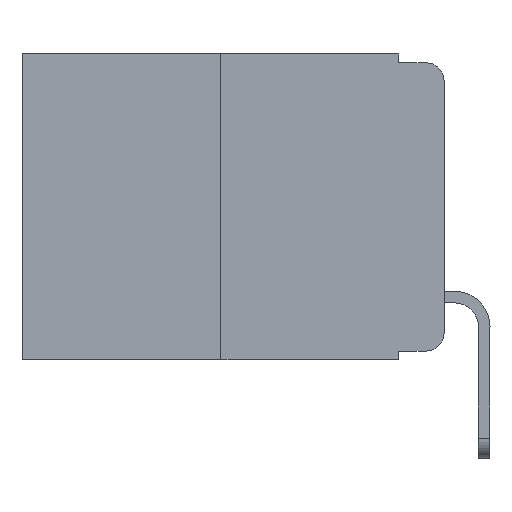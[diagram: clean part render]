
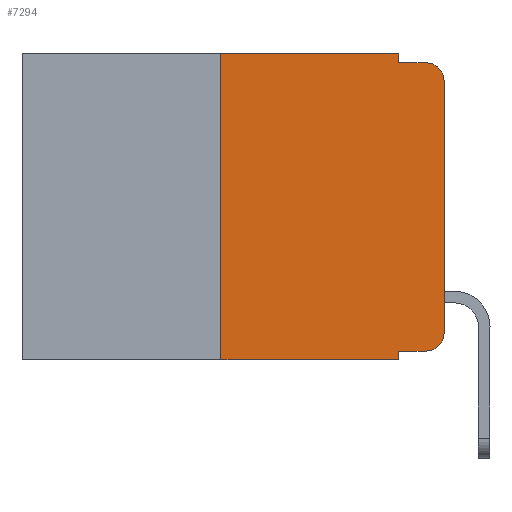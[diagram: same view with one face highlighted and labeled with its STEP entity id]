
A CAD part, left-side view. The second image highlights one B-rep face of the part: STEP entity #7294.
In plain terms, the highlighted planar face has unit normal (-1, 0, 0).
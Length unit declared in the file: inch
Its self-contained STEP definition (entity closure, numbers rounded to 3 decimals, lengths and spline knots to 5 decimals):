
#177 = ORIENTED_EDGE ( 'NONE', *, *, #3512, .F. ) ;
#372 = CARTESIAN_POINT ( 'NONE',  ( 0., 0.02, -0.01 ) ) ;
#486 = VECTOR ( 'NONE', #6335, 39.37008 ) ;
#684 = DIRECTION ( 'NONE',  ( 0., -1., 0. ) ) ;
#727 = FACE_OUTER_BOUND ( 'NONE', #8281, .T. ) ;
#996 = DIRECTION ( 'NONE',  ( 0., -1., 0. ) ) ;
#1347 = DIRECTION ( 'NONE',  ( 0., 0., -1. ) ) ;
#1359 = LINE ( 'NONE', #2402, #486 ) ;
#1383 = CARTESIAN_POINT ( 'NONE',  ( 0., 0.25, 0. ) ) ;
#1473 = VERTEX_POINT ( 'NONE', #8407 ) ;
#1579 = ORIENTED_EDGE ( 'NONE', *, *, #7550, .T. ) ;
#1868 = VERTEX_POINT ( 'NONE', #372 ) ;
#2193 = DIRECTION ( 'NONE',  ( -1., 0., 0. ) ) ;
#2281 = EDGE_CURVE ( 'NONE', #10485, #6231, #9210, .T. ) ;
#2402 = CARTESIAN_POINT ( 'NONE',  ( 0., 0., 0. ) ) ;
#2620 = CARTESIAN_POINT ( 'NONE',  ( 0., 0.473, 0. ) ) ;
#2724 = LINE ( 'NONE', #12498, #16344 ) ;
#2760 = VECTOR ( 'NONE', #1347, 39.37008 ) ;
#2765 = CARTESIAN_POINT ( 'NONE',  ( 0., 0., -0.03 ) ) ;
#2942 = EDGE_CURVE ( 'NONE', #6231, #13381, #16613, .T. ) ;
#3505 = PLANE ( 'NONE',  #12110 ) ;
#3512 = EDGE_CURVE ( 'NONE', #11973, #1473, #17265, .T. ) ;
#3532 = ORIENTED_EDGE ( 'NONE', *, *, #2281, .F. ) ;
#3641 = VERTEX_POINT ( 'NONE', #2765 ) ;
#4235 = LINE ( 'NONE', #4624, #17846 ) ;
#4285 = EDGE_CURVE ( 'NONE', #9864, #1473, #8345, .T. ) ;
#4324 = VERTEX_POINT ( 'NONE', #6524 ) ;
#4333 = DIRECTION ( 'NONE',  ( 0., 0., -1. ) ) ;
#4624 = CARTESIAN_POINT ( 'NONE',  ( 0., 0.051, -0.333 ) ) ;
#4796 = DIRECTION ( 'NONE',  ( 0., 0., -1. ) ) ;
#5360 = CARTESIAN_POINT ( 'NONE',  ( 0., 0.02, -0.333 ) ) ;
#5495 = EDGE_CURVE ( 'NONE', #13381, #1868, #2724, .T. ) ;
#6231 = VERTEX_POINT ( 'NONE', #14424 ) ;
#6335 = DIRECTION ( 'NONE',  ( 0., 0., 1. ) ) ;
#6524 = CARTESIAN_POINT ( 'NONE',  ( 0., 0., -0.313 ) ) ;
#6744 = EDGE_CURVE ( 'NONE', #4324, #3641, #1359, .T. ) ;
#7189 = EDGE_CURVE ( 'NONE', #16278, #4324, #17421, .T. ) ;
#7294 = ADVANCED_FACE ( 'NONE', ( #727 ), #3505, .F. ) ;
#7467 = VECTOR ( 'NONE', #996, 39.37008 ) ;
#7550 = EDGE_CURVE ( 'NONE', #11973, #16278, #4235, .T. ) ;
#7958 = DIRECTION ( 'NONE',  ( 1., 0., 0. ) ) ;
#8085 = CARTESIAN_POINT ( 'NONE',  ( 0., 0.473, 0. ) ) ;
#8281 = EDGE_LOOP ( 'NONE', ( #9598, #11539, #9960, #8879, #3532, #17536, #9479, #177, #1579, #11263 ) ) ;
#8345 = LINE ( 'NONE', #12111, #7467 ) ;
#8407 = CARTESIAN_POINT ( 'NONE',  ( 0., 0.051, -0.343 ) ) ;
#8674 = CARTESIAN_POINT ( 'NONE',  ( 0., 0.25, -0.343 ) ) ;
#8879 = ORIENTED_EDGE ( 'NONE', *, *, #2942, .F. ) ;
#8968 = CARTESIAN_POINT ( 'NONE',  ( 0., 0.051, -0.01 ) ) ;
#9114 = CARTESIAN_POINT ( 'NONE',  ( 0., 0.25, 0. ) ) ;
#9210 = LINE ( 'NONE', #2620, #10735 ) ;
#9240 = LINE ( 'NONE', #9114, #15804 ) ;
#9386 = EDGE_CURVE ( 'NONE', #9864, #10485, #9240, .T. ) ;
#9479 = ORIENTED_EDGE ( 'NONE', *, *, #4285, .T. ) ;
#9598 = ORIENTED_EDGE ( 'NONE', *, *, #6744, .T. ) ;
#9864 = VERTEX_POINT ( 'NONE', #8674 ) ;
#9955 = CARTESIAN_POINT ( 'NONE',  ( 0., 0.051, 0. ) ) ;
#9960 = ORIENTED_EDGE ( 'NONE', *, *, #5495, .F. ) ;
#10430 = DIRECTION ( 'NONE',  ( 0., 0., -1. ) ) ;
#10485 = VERTEX_POINT ( 'NONE', #1383 ) ;
#10735 = VECTOR ( 'NONE', #12513, 39.37008 ) ;
#11153 = DIRECTION ( 'NONE',  ( 0., -1., 0. ) ) ;
#11263 = ORIENTED_EDGE ( 'NONE', *, *, #7189, .T. ) ;
#11315 = CARTESIAN_POINT ( 'NONE',  ( 0., 0.051, 0. ) ) ;
#11539 = ORIENTED_EDGE ( 'NONE', *, *, #15972, .T. ) ;
#11973 = VERTEX_POINT ( 'NONE', #15923 ) ;
#12110 = AXIS2_PLACEMENT_3D ( 'NONE', #8085, #7958, #17797 ) ;
#12111 = CARTESIAN_POINT ( 'NONE',  ( 0., 0.473, -0.343 ) ) ;
#12498 = CARTESIAN_POINT ( 'NONE',  ( 0., 0.051, -0.01 ) ) ;
#12513 = DIRECTION ( 'NONE',  ( 0., -1., 0. ) ) ;
#13106 = DIRECTION ( 'NONE',  ( 0., 0., 1. ) ) ;
#13381 = VERTEX_POINT ( 'NONE', #8968 ) ;
#13429 = AXIS2_PLACEMENT_3D ( 'NONE', #15873, #17299, #10430 ) ;
#14424 = CARTESIAN_POINT ( 'NONE',  ( 0., 0.051, 0. ) ) ;
#14561 = CARTESIAN_POINT ( 'NONE',  ( 0., 0.02, -0.313 ) ) ;
#15103 = VECTOR ( 'NONE', #4333, 39.37008 ) ;
#15804 = VECTOR ( 'NONE', #13106, 39.37008 ) ;
#15873 = CARTESIAN_POINT ( 'NONE',  ( 0., 0.02, -0.03 ) ) ;
#15923 = CARTESIAN_POINT ( 'NONE',  ( 0., 0.051, -0.333 ) ) ;
#15972 = EDGE_CURVE ( 'NONE', #3641, #1868, #17053, .T. ) ;
#16278 = VERTEX_POINT ( 'NONE', #5360 ) ;
#16344 = VECTOR ( 'NONE', #11153, 39.37008 ) ;
#16613 = LINE ( 'NONE', #11315, #15103 ) ;
#17053 = CIRCLE ( 'NONE', #13429, 0.02 ) ;
#17265 = LINE ( 'NONE', #9955, #2760 ) ;
#17299 = DIRECTION ( 'NONE',  ( -1., 0., 0. ) ) ;
#17421 = CIRCLE ( 'NONE', #18006, 0.02 ) ;
#17536 = ORIENTED_EDGE ( 'NONE', *, *, #9386, .F. ) ;
#17797 = DIRECTION ( 'NONE',  ( 0., 0., -1. ) ) ;
#17846 = VECTOR ( 'NONE', #684, 39.37008 ) ;
#18006 = AXIS2_PLACEMENT_3D ( 'NONE', #14561, #2193, #4796 ) ;
